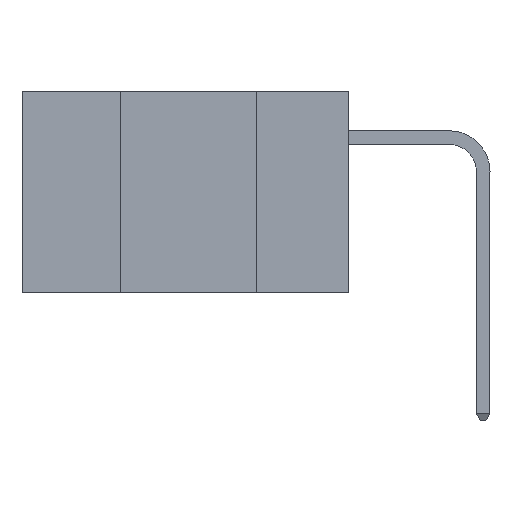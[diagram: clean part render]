
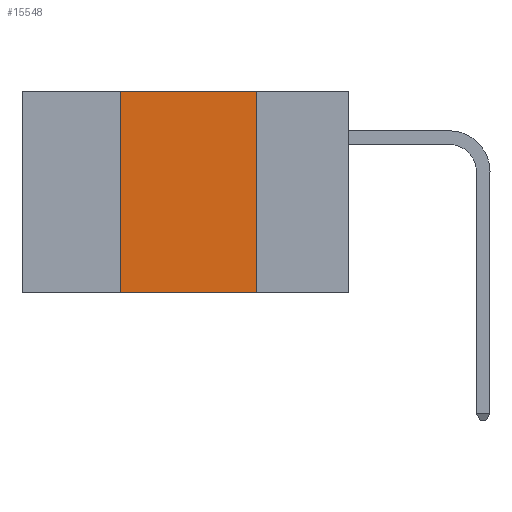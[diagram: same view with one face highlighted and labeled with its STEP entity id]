
A CAD part, left-side view. The second image highlights one B-rep face of the part: STEP entity #15548.
In plain terms, the highlighted planar face has unit normal (-1, 0, 0).
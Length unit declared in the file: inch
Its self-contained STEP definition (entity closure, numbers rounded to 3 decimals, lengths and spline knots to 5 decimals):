
#411 = CARTESIAN_POINT ( 'NONE',  ( 0., 0.17, -0.37 ) ) ;
#1780 = EDGE_CURVE ( 'NONE', #15106, #7865, #26550, .T. ) ;
#2597 = AXIS2_PLACEMENT_3D ( 'NONE', #25345, #9478, #7286 ) ;
#3277 = DIRECTION ( 'NONE',  ( 0., -1., 0. ) ) ;
#4198 = ORIENTED_EDGE ( 'NONE', *, *, #8148, .F. ) ;
#4230 = VERTEX_POINT ( 'NONE', #11480 ) ;
#5608 = VECTOR ( 'NONE', #24939, 39.37008 ) ;
#5861 = CARTESIAN_POINT ( 'NONE',  ( 0., 0.17, 0. ) ) ;
#6491 = VERTEX_POINT ( 'NONE', #15065 ) ;
#6525 = EDGE_CURVE ( 'NONE', #15106, #4230, #25965, .T. ) ;
#7286 = DIRECTION ( 'NONE',  ( 0., 0., -1. ) ) ;
#7865 = VERTEX_POINT ( 'NONE', #411 ) ;
#8148 = EDGE_CURVE ( 'NONE', #4230, #6491, #30272, .T. ) ;
#8466 = ORIENTED_EDGE ( 'NONE', *, *, #1780, .T. ) ;
#8856 = PLANE ( 'NONE',  #2597 ) ;
#9478 = DIRECTION ( 'NONE',  ( 1., 0., 0. ) ) ;
#10590 = FACE_OUTER_BOUND ( 'NONE', #29098, .T. ) ;
#11480 = CARTESIAN_POINT ( 'NONE',  ( 0., 0.42, 0. ) ) ;
#12973 = CARTESIAN_POINT ( 'NONE',  ( 0., 0.42, 0. ) ) ;
#15065 = CARTESIAN_POINT ( 'NONE',  ( 0., 0.17, 0. ) ) ;
#15106 = VERTEX_POINT ( 'NONE', #24424 ) ;
#15548 = ADVANCED_FACE ( 'NONE', ( #10590 ), #8856, .F. ) ;
#15603 = DIRECTION ( 'NONE',  ( 0., -1., 0. ) ) ;
#17672 = EDGE_CURVE ( 'NONE', #6491, #7865, #18220, .T. ) ;
#17730 = DIRECTION ( 'NONE',  ( 0., 0., 1. ) ) ;
#18220 = LINE ( 'NONE', #5861, #5608 ) ;
#19012 = VECTOR ( 'NONE', #17730, 39.37008 ) ;
#19675 = ORIENTED_EDGE ( 'NONE', *, *, #6525, .F. ) ;
#22109 = VECTOR ( 'NONE', #3277, 39.37008 ) ;
#24424 = CARTESIAN_POINT ( 'NONE',  ( 0., 0.42, -0.37 ) ) ;
#24500 = CARTESIAN_POINT ( 'NONE',  ( 0., 0.6, -0.37 ) ) ;
#24939 = DIRECTION ( 'NONE',  ( 0., 0., -1. ) ) ;
#25345 = CARTESIAN_POINT ( 'NONE',  ( 0., 0.6, 0. ) ) ;
#25965 = LINE ( 'NONE', #12973, #19012 ) ;
#26550 = LINE ( 'NONE', #24500, #22109 ) ;
#29098 = EDGE_LOOP ( 'NONE', ( #30379, #4198, #19675, #8466 ) ) ;
#29162 = VECTOR ( 'NONE', #15603, 39.37008 ) ;
#29462 = CARTESIAN_POINT ( 'NONE',  ( 0., 0.6, 0. ) ) ;
#30272 = LINE ( 'NONE', #29462, #29162 ) ;
#30379 = ORIENTED_EDGE ( 'NONE', *, *, #17672, .F. ) ;
